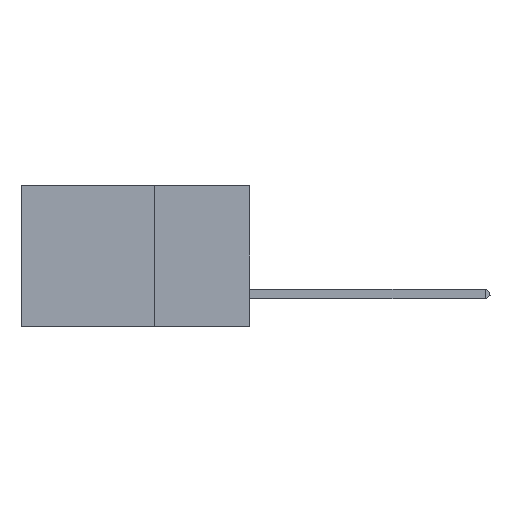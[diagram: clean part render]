
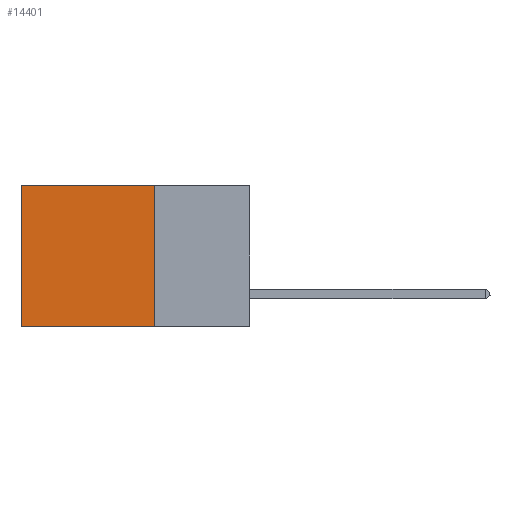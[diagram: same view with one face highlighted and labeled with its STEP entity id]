
A CAD part, left-side view. The second image highlights one B-rep face of the part: STEP entity #14401.
In plain terms, the highlighted planar face has unit normal (-1, 0, 0).
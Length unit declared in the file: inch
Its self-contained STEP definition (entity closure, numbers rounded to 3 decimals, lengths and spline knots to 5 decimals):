
#868 = CARTESIAN_POINT ( 'NONE',  ( 0.2875, 0.25, -0.37 ) ) ;
#2681 = DIRECTION ( 'NONE',  ( 1., 0., 0. ) ) ;
#3698 = ORIENTED_EDGE ( 'NONE', *, *, #6167, .T. ) ;
#4437 = VERTEX_POINT ( 'NONE', #5150 ) ;
#5150 = CARTESIAN_POINT ( 'NONE',  ( 0.2875, 0.6, -0.37 ) ) ;
#5202 = DIRECTION ( 'NONE',  ( 0., 0., -1. ) ) ;
#5823 = LINE ( 'NONE', #868, #20590 ) ;
#6167 = EDGE_CURVE ( 'NONE', #14219, #4437, #21935, .T. ) ;
#6283 = ORIENTED_EDGE ( 'NONE', *, *, #18201, .F. ) ;
#6575 = CARTESIAN_POINT ( 'NONE',  ( 0.2875, 0.25, 0. ) ) ;
#7251 = LINE ( 'NONE', #13969, #7797 ) ;
#7708 = CARTESIAN_POINT ( 'NONE',  ( 0.2875, 0.6, 0. ) ) ;
#7797 = VECTOR ( 'NONE', #17196, 39.37008 ) ;
#7873 = DIRECTION ( 'NONE',  ( 0., 0., -1. ) ) ;
#8563 = CARTESIAN_POINT ( 'NONE',  ( 0.2875, 0.6, 0. ) ) ;
#9409 = EDGE_CURVE ( 'NONE', #22171, #14219, #7251, .T. ) ;
#9908 = EDGE_CURVE ( 'NONE', #12977, #4437, #5823, .T. ) ;
#10422 = VECTOR ( 'NONE', #13439, 39.37008 ) ;
#12369 = CARTESIAN_POINT ( 'NONE',  ( 0.2875, 0.25, -0.37 ) ) ;
#12811 = VECTOR ( 'NONE', #5202, 39.37008 ) ;
#12977 = VERTEX_POINT ( 'NONE', #12369 ) ;
#13439 = DIRECTION ( 'NONE',  ( 0., 0., -1. ) ) ;
#13763 = ORIENTED_EDGE ( 'NONE', *, *, #9908, .F. ) ;
#13969 = CARTESIAN_POINT ( 'NONE',  ( 0.2875, 0.25, 0. ) ) ;
#14219 = VERTEX_POINT ( 'NONE', #7708 ) ;
#14401 = ADVANCED_FACE ( 'NONE', ( #17856 ), #21526, .F. ) ;
#14483 = ORIENTED_EDGE ( 'NONE', *, *, #9409, .T. ) ;
#14666 = DIRECTION ( 'NONE',  ( 0., 1., 0. ) ) ;
#14879 = CARTESIAN_POINT ( 'NONE',  ( 0.2875, 0.25, 0. ) ) ;
#15293 = LINE ( 'NONE', #6575, #10422 ) ;
#15516 = AXIS2_PLACEMENT_3D ( 'NONE', #14879, #2681, #7873 ) ;
#17196 = DIRECTION ( 'NONE',  ( 0., 1., 0. ) ) ;
#17856 = FACE_OUTER_BOUND ( 'NONE', #18628, .T. ) ;
#18201 = EDGE_CURVE ( 'NONE', #22171, #12977, #15293, .T. ) ;
#18628 = EDGE_LOOP ( 'NONE', ( #3698, #13763, #6283, #14483 ) ) ;
#20590 = VECTOR ( 'NONE', #14666, 39.37008 ) ;
#20714 = CARTESIAN_POINT ( 'NONE',  ( 0.2875, 0.25, 0. ) ) ;
#21526 = PLANE ( 'NONE',  #15516 ) ;
#21935 = LINE ( 'NONE', #8563, #12811 ) ;
#22171 = VERTEX_POINT ( 'NONE', #20714 ) ;
